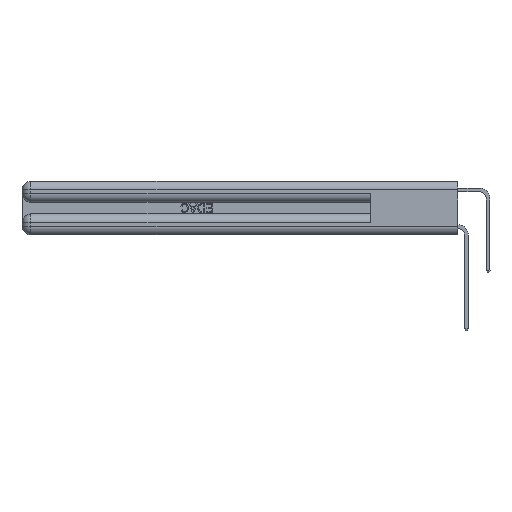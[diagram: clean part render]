
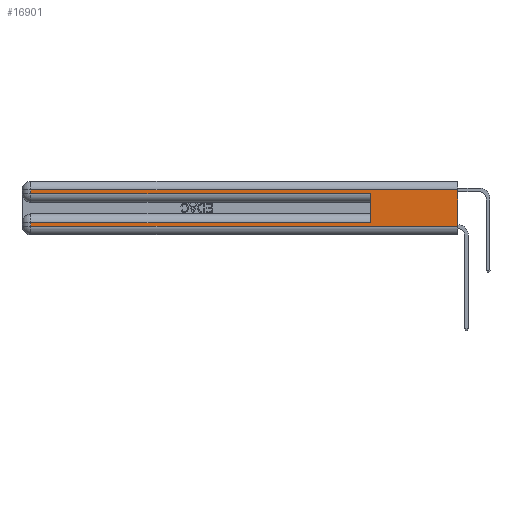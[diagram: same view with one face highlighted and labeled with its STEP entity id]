
A CAD part, left-side view. The second image highlights one B-rep face of the part: STEP entity #16901.
In plain terms, the highlighted planar face has unit normal (-1, 0, 0).
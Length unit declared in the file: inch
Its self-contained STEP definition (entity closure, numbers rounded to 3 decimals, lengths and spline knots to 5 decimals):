
#135 = CARTESIAN_POINT ( 'NONE',  ( 0., 0., 0.37 ) ) ;
#224 = VERTEX_POINT ( 'NONE', #15174 ) ;
#715 = LINE ( 'NONE', #8495, #21795 ) ;
#1569 = VERTEX_POINT ( 'NONE', #25972 ) ;
#1811 = AXIS2_PLACEMENT_3D ( 'NONE', #3586, #24490, #16193 ) ;
#1881 = DIRECTION ( 'NONE',  ( 0., 0., 1. ) ) ;
#1908 = EDGE_CURVE ( 'NONE', #31222, #24068, #14473, .T. ) ;
#3358 = DIRECTION ( 'NONE',  ( 0., 1., 0. ) ) ;
#3586 = CARTESIAN_POINT ( 'NONE',  ( 0., 0., 0.37 ) ) ;
#3964 = EDGE_CURVE ( 'NONE', #224, #20960, #7590, .T. ) ;
#4093 = ORIENTED_EDGE ( 'NONE', *, *, #19853, .T. ) ;
#5582 = CARTESIAN_POINT ( 'NONE',  ( 0., 2.94, 0.085 ) ) ;
#6721 = FACE_OUTER_BOUND ( 'NONE', #29841, .T. ) ;
#7004 = DIRECTION ( 'NONE',  ( 0., 0., -1. ) ) ;
#7368 = ORIENTED_EDGE ( 'NONE', *, *, #12879, .T. ) ;
#7590 = LINE ( 'NONE', #135, #19445 ) ;
#8400 = CARTESIAN_POINT ( 'NONE',  ( 0., 0., 0.06 ) ) ;
#8495 = CARTESIAN_POINT ( 'NONE',  ( 0., 0., 0.31 ) ) ;
#8969 = ORIENTED_EDGE ( 'NONE', *, *, #1908, .F. ) ;
#10231 = DIRECTION ( 'NONE',  ( 0., 0., -1. ) ) ;
#10874 = LINE ( 'NONE', #8400, #12301 ) ;
#11636 = CARTESIAN_POINT ( 'NONE',  ( 0., 2.94, 0.37 ) ) ;
#12149 = VECTOR ( 'NONE', #17275, 39.37008 ) ;
#12301 = VECTOR ( 'NONE', #23835, 39.37008 ) ;
#12764 = CARTESIAN_POINT ( 'NONE',  ( 0., 2.94, 0.31 ) ) ;
#12879 = EDGE_CURVE ( 'NONE', #18806, #20960, #10874, .T. ) ;
#13062 = VECTOR ( 'NONE', #21791, 39.37008 ) ;
#13837 = VERTEX_POINT ( 'NONE', #12764 ) ;
#13977 = ORIENTED_EDGE ( 'NONE', *, *, #22243, .T. ) ;
#14473 = LINE ( 'NONE', #17151, #22877 ) ;
#14521 = ORIENTED_EDGE ( 'NONE', *, *, #32262, .T. ) ;
#14894 = LINE ( 'NONE', #16902, #31628 ) ;
#15174 = CARTESIAN_POINT ( 'NONE',  ( 0., 0., 0.31 ) ) ;
#16193 = DIRECTION ( 'NONE',  ( 0., 0., -1. ) ) ;
#16786 = ORIENTED_EDGE ( 'NONE', *, *, #22388, .T. ) ;
#16865 = VERTEX_POINT ( 'NONE', #5582 ) ;
#16901 = ADVANCED_FACE ( 'NONE', ( #6721 ), #31464, .F. ) ;
#16902 = CARTESIAN_POINT ( 'NONE',  ( 0., 0., 0.085 ) ) ;
#17151 = CARTESIAN_POINT ( 'NONE',  ( 0., 0.6, 0.145 ) ) ;
#17275 = DIRECTION ( 'NONE',  ( 0., -1., 0. ) ) ;
#17399 = CARTESIAN_POINT ( 'NONE',  ( 0., 0.6, 0.085 ) ) ;
#18806 = VERTEX_POINT ( 'NONE', #28766 ) ;
#19445 = VECTOR ( 'NONE', #10231, 39.37008 ) ;
#19853 = EDGE_CURVE ( 'NONE', #31222, #16865, #14894, .T. ) ;
#20960 = VERTEX_POINT ( 'NONE', #29394 ) ;
#21081 = ORIENTED_EDGE ( 'NONE', *, *, #30676, .T. ) ;
#21791 = DIRECTION ( 'NONE',  ( 0., 0., -1. ) ) ;
#21795 = VECTOR ( 'NONE', #3358, 39.37008 ) ;
#22243 = EDGE_CURVE ( 'NONE', #16865, #18806, #24270, .T. ) ;
#22259 = LINE ( 'NONE', #32367, #12149 ) ;
#22323 = ORIENTED_EDGE ( 'NONE', *, *, #3964, .F. ) ;
#22388 = EDGE_CURVE ( 'NONE', #13837, #1569, #32069, .T. ) ;
#22877 = VECTOR ( 'NONE', #1881, 39.37008 ) ;
#23835 = DIRECTION ( 'NONE',  ( 0., -1., 0. ) ) ;
#24068 = VERTEX_POINT ( 'NONE', #29868 ) ;
#24270 = LINE ( 'NONE', #11636, #13062 ) ;
#24490 = DIRECTION ( 'NONE',  ( 1., 0., 0. ) ) ;
#24877 = DIRECTION ( 'NONE',  ( 0., 1., 0. ) ) ;
#25972 = CARTESIAN_POINT ( 'NONE',  ( 0., 2.94, 0.285 ) ) ;
#26895 = VECTOR ( 'NONE', #7004, 39.37008 ) ;
#28766 = CARTESIAN_POINT ( 'NONE',  ( 0., 2.94, 0.06 ) ) ;
#29394 = CARTESIAN_POINT ( 'NONE',  ( 0., 0., 0.06 ) ) ;
#29731 = CARTESIAN_POINT ( 'NONE',  ( 0., 2.94, 0.37 ) ) ;
#29841 = EDGE_LOOP ( 'NONE', ( #22323, #14521, #16786, #21081, #8969, #4093, #13977, #7368 ) ) ;
#29868 = CARTESIAN_POINT ( 'NONE',  ( 0., 0.6, 0.285 ) ) ;
#30676 = EDGE_CURVE ( 'NONE', #1569, #24068, #22259, .T. ) ;
#31222 = VERTEX_POINT ( 'NONE', #17399 ) ;
#31464 = PLANE ( 'NONE',  #1811 ) ;
#31628 = VECTOR ( 'NONE', #24877, 39.37008 ) ;
#32069 = LINE ( 'NONE', #29731, #26895 ) ;
#32262 = EDGE_CURVE ( 'NONE', #224, #13837, #715, .T. ) ;
#32367 = CARTESIAN_POINT ( 'NONE',  ( 0., 0., 0.285 ) ) ;
